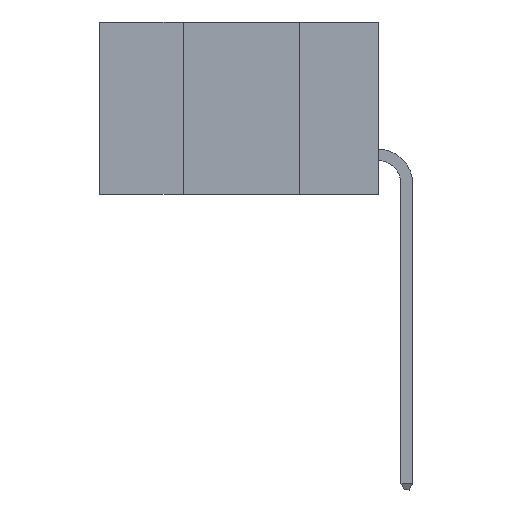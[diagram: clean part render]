
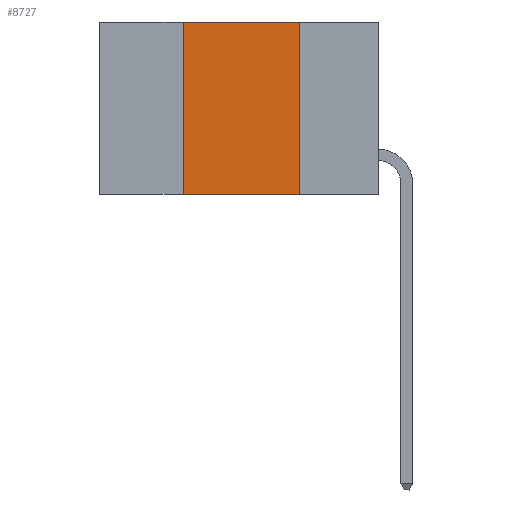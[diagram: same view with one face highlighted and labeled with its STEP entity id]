
A CAD part, left-side view. The second image highlights one B-rep face of the part: STEP entity #8727.
In plain terms, the highlighted planar face has unit normal (-1, 0, 0).
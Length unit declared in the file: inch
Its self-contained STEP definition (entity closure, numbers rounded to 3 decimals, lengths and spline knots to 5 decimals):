
#535 = EDGE_CURVE ( 'NONE', #7732, #1380, #6700, .T. ) ;
#764 = AXIS2_PLACEMENT_3D ( 'NONE', #3238, #2979, #800 ) ;
#791 = VERTEX_POINT ( 'NONE', #8887 ) ;
#800 = DIRECTION ( 'NONE',  ( 0., 0., -1. ) ) ;
#1380 = VERTEX_POINT ( 'NONE', #9576 ) ;
#2423 = VERTEX_POINT ( 'NONE', #4715 ) ;
#2487 = ORIENTED_EDGE ( 'NONE', *, *, #6060, .F. ) ;
#2979 = DIRECTION ( 'NONE',  ( 1., 0., 0. ) ) ;
#3120 = DIRECTION ( 'NONE',  ( 0., 0., 1. ) ) ;
#3238 = CARTESIAN_POINT ( 'NONE',  ( 0., 0.6, 0. ) ) ;
#3395 = ORIENTED_EDGE ( 'NONE', *, *, #535, .F. ) ;
#3707 = EDGE_LOOP ( 'NONE', ( #2487, #7533, #3395, #7075 ) ) ;
#3837 = CARTESIAN_POINT ( 'NONE',  ( 0., 0.6, -0.37 ) ) ;
#3931 = DIRECTION ( 'NONE',  ( 0., 0., -1. ) ) ;
#4191 = CARTESIAN_POINT ( 'NONE',  ( 0., 0.42, -0.37 ) ) ;
#4418 = CARTESIAN_POINT ( 'NONE',  ( 0., 0.17, 0. ) ) ;
#4715 = CARTESIAN_POINT ( 'NONE',  ( 0., 0.17, 0. ) ) ;
#5294 = DIRECTION ( 'NONE',  ( 0., -1., 0. ) ) ;
#5363 = VECTOR ( 'NONE', #3931, 39.37008 ) ;
#5457 = VECTOR ( 'NONE', #5294, 39.37008 ) ;
#5649 = FACE_OUTER_BOUND ( 'NONE', #3707, .T. ) ;
#6060 = EDGE_CURVE ( 'NONE', #2423, #791, #8950, .T. ) ;
#6606 = EDGE_CURVE ( 'NONE', #7732, #791, #9646, .T. ) ;
#6700 = LINE ( 'NONE', #7992, #7163 ) ;
#6773 = CARTESIAN_POINT ( 'NONE',  ( 0., 0.6, 0. ) ) ;
#7060 = EDGE_CURVE ( 'NONE', #1380, #2423, #7840, .T. ) ;
#7075 = ORIENTED_EDGE ( 'NONE', *, *, #6606, .T. ) ;
#7163 = VECTOR ( 'NONE', #3120, 39.37008 ) ;
#7533 = ORIENTED_EDGE ( 'NONE', *, *, #7060, .F. ) ;
#7732 = VERTEX_POINT ( 'NONE', #4191 ) ;
#7840 = LINE ( 'NONE', #6773, #5457 ) ;
#7848 = VECTOR ( 'NONE', #8238, 39.37008 ) ;
#7992 = CARTESIAN_POINT ( 'NONE',  ( 0., 0.42, 0. ) ) ;
#8238 = DIRECTION ( 'NONE',  ( 0., -1., 0. ) ) ;
#8727 = ADVANCED_FACE ( 'NONE', ( #5649 ), #9277, .F. ) ;
#8887 = CARTESIAN_POINT ( 'NONE',  ( 0., 0.17, -0.37 ) ) ;
#8950 = LINE ( 'NONE', #4418, #5363 ) ;
#9277 = PLANE ( 'NONE',  #764 ) ;
#9576 = CARTESIAN_POINT ( 'NONE',  ( 0., 0.42, 0. ) ) ;
#9646 = LINE ( 'NONE', #3837, #7848 ) ;
